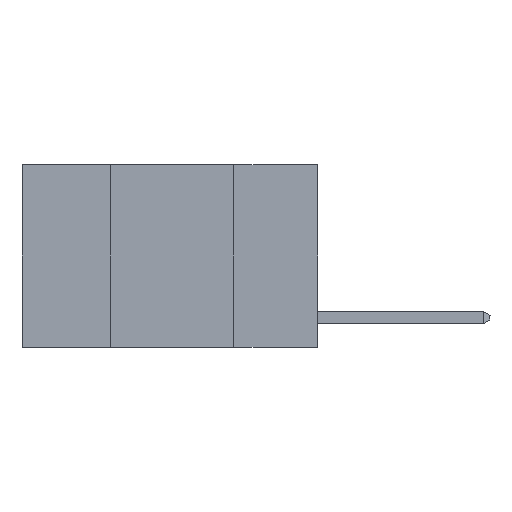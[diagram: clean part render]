
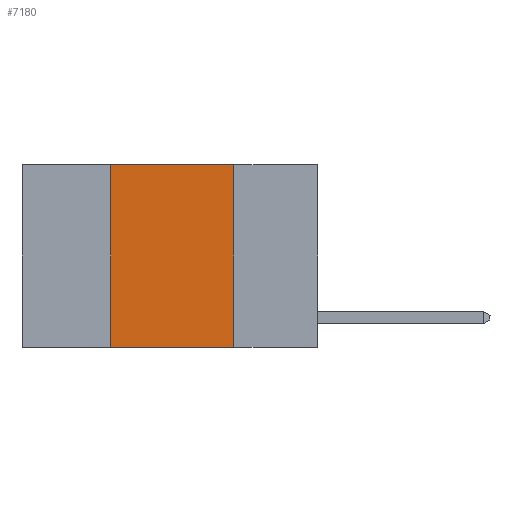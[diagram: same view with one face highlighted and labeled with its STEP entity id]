
A CAD part, left-side view. The second image highlights one B-rep face of the part: STEP entity #7180.
In plain terms, the highlighted planar face has unit normal (-1, 0, 0).
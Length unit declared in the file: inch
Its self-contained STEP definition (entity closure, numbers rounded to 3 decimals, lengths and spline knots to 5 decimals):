
#881 = VECTOR ( 'NONE', #4495, 39.37008 ) ;
#1087 = CARTESIAN_POINT ( 'NONE',  ( 0., 0.42, -0.37 ) ) ;
#2289 = VECTOR ( 'NONE', #16821, 39.37008 ) ;
#2354 = LINE ( 'NONE', #19626, #7025 ) ;
#3540 = LINE ( 'NONE', #13069, #2289 ) ;
#4412 = DIRECTION ( 'NONE',  ( 0., -1., 0. ) ) ;
#4495 = DIRECTION ( 'NONE',  ( 0., 0., 1. ) ) ;
#5520 = DIRECTION ( 'NONE',  ( 0., 0., -1. ) ) ;
#7025 = VECTOR ( 'NONE', #9982, 39.37008 ) ;
#7180 = ADVANCED_FACE ( 'NONE', ( #18963 ), #22671, .F. ) ;
#7200 = EDGE_CURVE ( 'NONE', #18275, #11423, #3540, .T. ) ;
#8590 = EDGE_CURVE ( 'NONE', #10265, #11423, #2354, .T. ) ;
#9982 = DIRECTION ( 'NONE',  ( 0., 0., -1. ) ) ;
#10265 = VERTEX_POINT ( 'NONE', #10306 ) ;
#10306 = CARTESIAN_POINT ( 'NONE',  ( 0., 0.17, 0. ) ) ;
#11194 = EDGE_CURVE ( 'NONE', #20608, #10265, #21428, .T. ) ;
#11423 = VERTEX_POINT ( 'NONE', #23398 ) ;
#12268 = ORIENTED_EDGE ( 'NONE', *, *, #17646, .F. ) ;
#12817 = ORIENTED_EDGE ( 'NONE', *, *, #11194, .F. ) ;
#13069 = CARTESIAN_POINT ( 'NONE',  ( 0., 0.6, -0.37 ) ) ;
#14064 = ORIENTED_EDGE ( 'NONE', *, *, #8590, .F. ) ;
#15322 = CARTESIAN_POINT ( 'NONE',  ( 0., 0.6, 0. ) ) ;
#15806 = LINE ( 'NONE', #23394, #881 ) ;
#16821 = DIRECTION ( 'NONE',  ( 0., -1., 0. ) ) ;
#17260 = CARTESIAN_POINT ( 'NONE',  ( 0., 0.42, 0. ) ) ;
#17646 = EDGE_CURVE ( 'NONE', #18275, #20608, #15806, .T. ) ;
#18068 = CARTESIAN_POINT ( 'NONE',  ( 0., 0.6, 0. ) ) ;
#18275 = VERTEX_POINT ( 'NONE', #1087 ) ;
#18562 = AXIS2_PLACEMENT_3D ( 'NONE', #15322, #22547, #5520 ) ;
#18963 = FACE_OUTER_BOUND ( 'NONE', #23758, .T. ) ;
#19626 = CARTESIAN_POINT ( 'NONE',  ( 0., 0.17, 0. ) ) ;
#20608 = VERTEX_POINT ( 'NONE', #17260 ) ;
#21428 = LINE ( 'NONE', #18068, #24221 ) ;
#22547 = DIRECTION ( 'NONE',  ( 1., 0., 0. ) ) ;
#22671 = PLANE ( 'NONE',  #18562 ) ;
#23394 = CARTESIAN_POINT ( 'NONE',  ( 0., 0.42, 0. ) ) ;
#23398 = CARTESIAN_POINT ( 'NONE',  ( 0., 0.17, -0.37 ) ) ;
#23758 = EDGE_LOOP ( 'NONE', ( #14064, #12817, #12268, #24408 ) ) ;
#24221 = VECTOR ( 'NONE', #4412, 39.37008 ) ;
#24408 = ORIENTED_EDGE ( 'NONE', *, *, #7200, .T. ) ;
